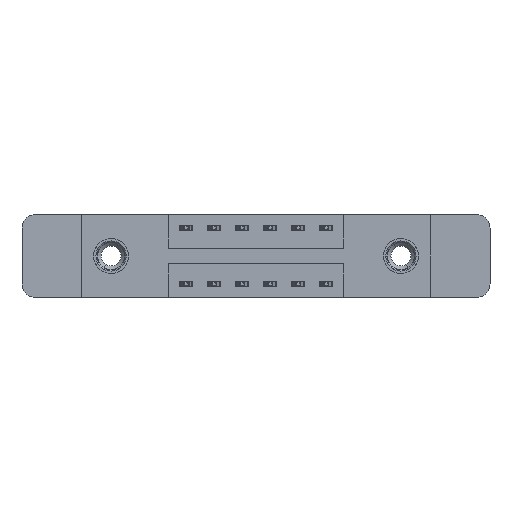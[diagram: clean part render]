
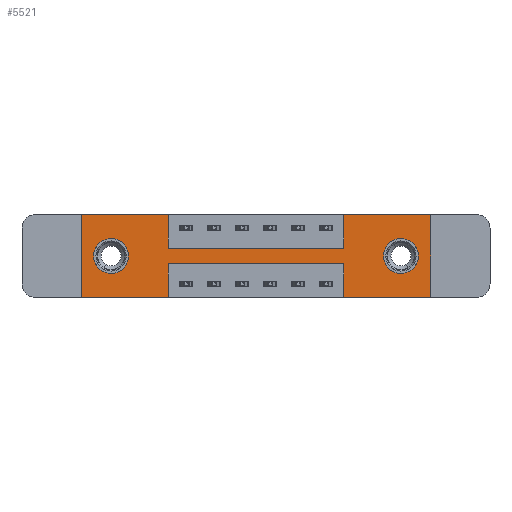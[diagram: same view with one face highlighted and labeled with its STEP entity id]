
A CAD part, front view. The second image highlights one B-rep face of the part: STEP entity #5521.
In plain terms, the highlighted planar face has unit normal (0, -1, 0).
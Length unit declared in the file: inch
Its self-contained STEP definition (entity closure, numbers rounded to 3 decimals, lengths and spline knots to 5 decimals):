
#49 = CARTESIAN_POINT ( 'NONE',  ( 0., 0., 0. ) ) ;
#125 = CARTESIAN_POINT ( 'NONE',  ( 0., 0., -0.37 ) ) ;
#145 = DIRECTION ( 'NONE',  ( 0., 0., -1. ) ) ;
#163 = EDGE_CURVE ( 'NONE', #9254, #5198, #9706, .T. ) ;
#224 = EDGE_CURVE ( 'NONE', #13569, #11813, #9871, .T. ) ;
#245 = AXIS2_PLACEMENT_3D ( 'NONE', #5543, #1392, #11990 ) ;
#277 = CARTESIAN_POINT ( 'NONE',  ( 0.3875, 0., 0. ) ) ;
#530 = VECTOR ( 'NONE', #6954, 39.37008 ) ;
#551 = EDGE_CURVE ( 'NONE', #3224, #10590, #8332, .T. ) ;
#721 = DIRECTION ( 'NONE',  ( 0., 0., -1. ) ) ;
#783 = EDGE_CURVE ( 'NONE', #13189, #3225, #10357, .T. ) ;
#973 = ORIENTED_EDGE ( 'NONE', *, *, #6170, .F. ) ;
#1083 = VERTEX_POINT ( 'NONE', #7836 ) ;
#1301 = CARTESIAN_POINT ( 'NONE',  ( 0., 0., 0. ) ) ;
#1333 = LINE ( 'NONE', #11857, #8520 ) ;
#1392 = DIRECTION ( 'NONE',  ( 0., 1., 0. ) ) ;
#1503 = LINE ( 'NONE', #8303, #12790 ) ;
#1569 = ORIENTED_EDGE ( 'NONE', *, *, #6031, .T. ) ;
#1575 = FACE_BOUND ( 'NONE', #7010, .T. ) ;
#1605 = DIRECTION ( 'NONE',  ( 0., 0., 1. ) ) ;
#1612 = LINE ( 'NONE', #13269, #10345 ) ;
#1788 = EDGE_CURVE ( 'NONE', #7547, #7026, #9482, .T. ) ;
#1999 = EDGE_CURVE ( 'NONE', #7026, #6570, #2979, .T. ) ;
#2111 = DIRECTION ( 'NONE',  ( -1., 0., 0. ) ) ;
#2160 = EDGE_CURVE ( 'NONE', #10590, #1083, #1612, .T. ) ;
#2506 = CARTESIAN_POINT ( 'NONE',  ( 1.4275, 0., -0.185 ) ) ;
#2564 = CARTESIAN_POINT ( 'NONE',  ( 0., 0., -0.37 ) ) ;
#2616 = CARTESIAN_POINT ( 'NONE',  ( 0.3875, 0., -0.37 ) ) ;
#2861 = ORIENTED_EDGE ( 'NONE', *, *, #551, .F. ) ;
#2963 = CARTESIAN_POINT ( 'NONE',  ( 0.3875, 0., -0.22 ) ) ;
#2979 = LINE ( 'NONE', #4013, #9153 ) ;
#3224 = VERTEX_POINT ( 'NONE', #9418 ) ;
#3225 = VERTEX_POINT ( 'NONE', #4147 ) ;
#3241 = DIRECTION ( 'NONE',  ( 0., 0., 1. ) ) ;
#3264 = VERTEX_POINT ( 'NONE', #13984 ) ;
#3434 = VERTEX_POINT ( 'NONE', #8209 ) ;
#3505 = EDGE_LOOP ( 'NONE', ( #13092, #13299, #4454, #12283, #13648, #13823, #7395, #2861, #973, #12263, #9962, #4703 ) ) ;
#3510 = ORIENTED_EDGE ( 'NONE', *, *, #5349, .T. ) ;
#3531 = LINE ( 'NONE', #277, #4208 ) ;
#3712 = CIRCLE ( 'NONE', #11984, 0.078 ) ;
#3809 = CARTESIAN_POINT ( 'NONE',  ( 1.56, 0., 0. ) ) ;
#3938 = CARTESIAN_POINT ( 'NONE',  ( 1.4275, 0., -0.107 ) ) ;
#4013 = CARTESIAN_POINT ( 'NONE',  ( 0.3875, 0., -0.37 ) ) ;
#4147 = CARTESIAN_POINT ( 'NONE',  ( 0.1325, 0., -0.107 ) ) ;
#4208 = VECTOR ( 'NONE', #145, 39.37008 ) ;
#4216 = CARTESIAN_POINT ( 'NONE',  ( 0.1325, 0., -0.185 ) ) ;
#4347 = EDGE_CURVE ( 'NONE', #1083, #13569, #6209, .T. ) ;
#4438 = CARTESIAN_POINT ( 'NONE',  ( 0., 0., -0.37 ) ) ;
#4454 = ORIENTED_EDGE ( 'NONE', *, *, #8108, .F. ) ;
#4703 = ORIENTED_EDGE ( 'NONE', *, *, #11196, .F. ) ;
#4974 = DIRECTION ( 'NONE',  ( 0., 0., -1. ) ) ;
#4976 = VERTEX_POINT ( 'NONE', #125 ) ;
#5198 = VERTEX_POINT ( 'NONE', #6882 ) ;
#5349 = EDGE_CURVE ( 'NONE', #12794, #3264, #3712, .T. ) ;
#5521 = ADVANCED_FACE ( 'NONE', ( #13868, #1575, #6751 ), #13564, .T. ) ;
#5543 = CARTESIAN_POINT ( 'NONE',  ( 0.1325, 0., -0.185 ) ) ;
#6031 = EDGE_CURVE ( 'NONE', #3225, #13189, #10446, .T. ) ;
#6041 = CARTESIAN_POINT ( 'NONE',  ( 0., 0., 0. ) ) ;
#6085 = DIRECTION ( 'NONE',  ( 0., 1., 0. ) ) ;
#6170 = EDGE_CURVE ( 'NONE', #5198, #3224, #3531, .T. ) ;
#6209 = LINE ( 'NONE', #1301, #530 ) ;
#6570 = VERTEX_POINT ( 'NONE', #2616 ) ;
#6751 = FACE_OUTER_BOUND ( 'NONE', #3505, .T. ) ;
#6882 = CARTESIAN_POINT ( 'NONE',  ( 0.3875, 0., 0. ) ) ;
#6924 = EDGE_CURVE ( 'NONE', #11813, #3434, #7732, .T. ) ;
#6954 = DIRECTION ( 'NONE',  ( 1., 0., 0. ) ) ;
#7010 = EDGE_LOOP ( 'NONE', ( #1569, #13214 ) ) ;
#7026 = VERTEX_POINT ( 'NONE', #11985 ) ;
#7105 = CARTESIAN_POINT ( 'NONE',  ( 1.4275, 0., -0.185 ) ) ;
#7395 = ORIENTED_EDGE ( 'NONE', *, *, #2160, .F. ) ;
#7461 = DIRECTION ( 'NONE',  ( 0., 1., 0. ) ) ;
#7518 = VECTOR ( 'NONE', #11770, 39.37008 ) ;
#7547 = VERTEX_POINT ( 'NONE', #10512 ) ;
#7668 = VECTOR ( 'NONE', #2111, 39.37008 ) ;
#7732 = LINE ( 'NONE', #4438, #12149 ) ;
#7836 = CARTESIAN_POINT ( 'NONE',  ( 1.1725, 0., 0. ) ) ;
#8047 = DIRECTION ( 'NONE',  ( 0., -1., 0. ) ) ;
#8075 = EDGE_CURVE ( 'NONE', #4976, #9254, #1503, .T. ) ;
#8108 = EDGE_CURVE ( 'NONE', #3434, #7547, #1333, .T. ) ;
#8209 = CARTESIAN_POINT ( 'NONE',  ( 1.1725, 0., -0.37 ) ) ;
#8301 = CARTESIAN_POINT ( 'NONE',  ( 0.1325, 0., -0.263 ) ) ;
#8303 = CARTESIAN_POINT ( 'NONE',  ( 0., 0., 0. ) ) ;
#8311 = DIRECTION ( 'NONE',  ( 0., 0., 1. ) ) ;
#8332 = LINE ( 'NONE', #9835, #9856 ) ;
#8366 = AXIS2_PLACEMENT_3D ( 'NONE', #2506, #9006, #9998 ) ;
#8520 = VECTOR ( 'NONE', #3241, 39.37008 ) ;
#8560 = CARTESIAN_POINT ( 'NONE',  ( 1.56, 0., 0. ) ) ;
#8810 = CARTESIAN_POINT ( 'NONE',  ( 1.56, 0., -0.37 ) ) ;
#8832 = DIRECTION ( 'NONE',  ( 1., 0., 0. ) ) ;
#8966 = VECTOR ( 'NONE', #9075, 39.37008 ) ;
#9006 = DIRECTION ( 'NONE',  ( 0., 1., 0. ) ) ;
#9075 = DIRECTION ( 'NONE',  ( -1., 0., 0. ) ) ;
#9153 = VECTOR ( 'NONE', #12683, 39.37008 ) ;
#9254 = VERTEX_POINT ( 'NONE', #6041 ) ;
#9297 = LINE ( 'NONE', #2564, #8966 ) ;
#9418 = CARTESIAN_POINT ( 'NONE',  ( 0.3875, 0., -0.15 ) ) ;
#9482 = LINE ( 'NONE', #2963, #7668 ) ;
#9666 = CARTESIAN_POINT ( 'NONE',  ( 1.1725, 0., -0.15 ) ) ;
#9706 = LINE ( 'NONE', #49, #7518 ) ;
#9835 = CARTESIAN_POINT ( 'NONE',  ( 0.3875, 0., -0.15 ) ) ;
#9856 = VECTOR ( 'NONE', #8832, 39.37008 ) ;
#9871 = LINE ( 'NONE', #3809, #12770 ) ;
#9962 = ORIENTED_EDGE ( 'NONE', *, *, #8075, .F. ) ;
#9998 = DIRECTION ( 'NONE',  ( 0., 0., -1. ) ) ;
#10231 = AXIS2_PLACEMENT_3D ( 'NONE', #4216, #7461, #8311 ) ;
#10345 = VECTOR ( 'NONE', #1605, 39.37008 ) ;
#10357 = CIRCLE ( 'NONE', #10231, 0.078 ) ;
#10446 = CIRCLE ( 'NONE', #245, 0.078 ) ;
#10512 = CARTESIAN_POINT ( 'NONE',  ( 1.1725, 0., -0.22 ) ) ;
#10590 = VERTEX_POINT ( 'NONE', #9666 ) ;
#10641 = EDGE_CURVE ( 'NONE', #3264, #12794, #13393, .T. ) ;
#10791 = AXIS2_PLACEMENT_3D ( 'NONE', #11265, #8047, #11214 ) ;
#10876 = DIRECTION ( 'NONE',  ( 0., 0., 1. ) ) ;
#11196 = EDGE_CURVE ( 'NONE', #6570, #4976, #9297, .T. ) ;
#11214 = DIRECTION ( 'NONE',  ( 0., 0., -1. ) ) ;
#11265 = CARTESIAN_POINT ( 'NONE',  ( 0., 0., -0.37 ) ) ;
#11530 = ORIENTED_EDGE ( 'NONE', *, *, #10641, .T. ) ;
#11770 = DIRECTION ( 'NONE',  ( 1., 0., 0. ) ) ;
#11813 = VERTEX_POINT ( 'NONE', #8810 ) ;
#11857 = CARTESIAN_POINT ( 'NONE',  ( 1.1725, 0., -0.37 ) ) ;
#11984 = AXIS2_PLACEMENT_3D ( 'NONE', #7105, #6085, #721 ) ;
#11985 = CARTESIAN_POINT ( 'NONE',  ( 0.3875, 0., -0.22 ) ) ;
#11990 = DIRECTION ( 'NONE',  ( 0., 0., 1. ) ) ;
#12017 = DIRECTION ( 'NONE',  ( -1., 0., 0. ) ) ;
#12149 = VECTOR ( 'NONE', #12017, 39.37008 ) ;
#12263 = ORIENTED_EDGE ( 'NONE', *, *, #163, .F. ) ;
#12283 = ORIENTED_EDGE ( 'NONE', *, *, #6924, .F. ) ;
#12683 = DIRECTION ( 'NONE',  ( 0., 0., -1. ) ) ;
#12770 = VECTOR ( 'NONE', #4974, 39.37008 ) ;
#12790 = VECTOR ( 'NONE', #10876, 39.37008 ) ;
#12794 = VERTEX_POINT ( 'NONE', #3938 ) ;
#13092 = ORIENTED_EDGE ( 'NONE', *, *, #1999, .F. ) ;
#13161 = EDGE_LOOP ( 'NONE', ( #3510, #11530 ) ) ;
#13189 = VERTEX_POINT ( 'NONE', #8301 ) ;
#13214 = ORIENTED_EDGE ( 'NONE', *, *, #783, .T. ) ;
#13269 = CARTESIAN_POINT ( 'NONE',  ( 1.1725, 0., 0. ) ) ;
#13299 = ORIENTED_EDGE ( 'NONE', *, *, #1788, .F. ) ;
#13393 = CIRCLE ( 'NONE', #8366, 0.078 ) ;
#13564 = PLANE ( 'NONE',  #10791 ) ;
#13569 = VERTEX_POINT ( 'NONE', #8560 ) ;
#13648 = ORIENTED_EDGE ( 'NONE', *, *, #224, .F. ) ;
#13823 = ORIENTED_EDGE ( 'NONE', *, *, #4347, .F. ) ;
#13868 = FACE_BOUND ( 'NONE', #13161, .T. ) ;
#13984 = CARTESIAN_POINT ( 'NONE',  ( 1.4275, 0., -0.263 ) ) ;
